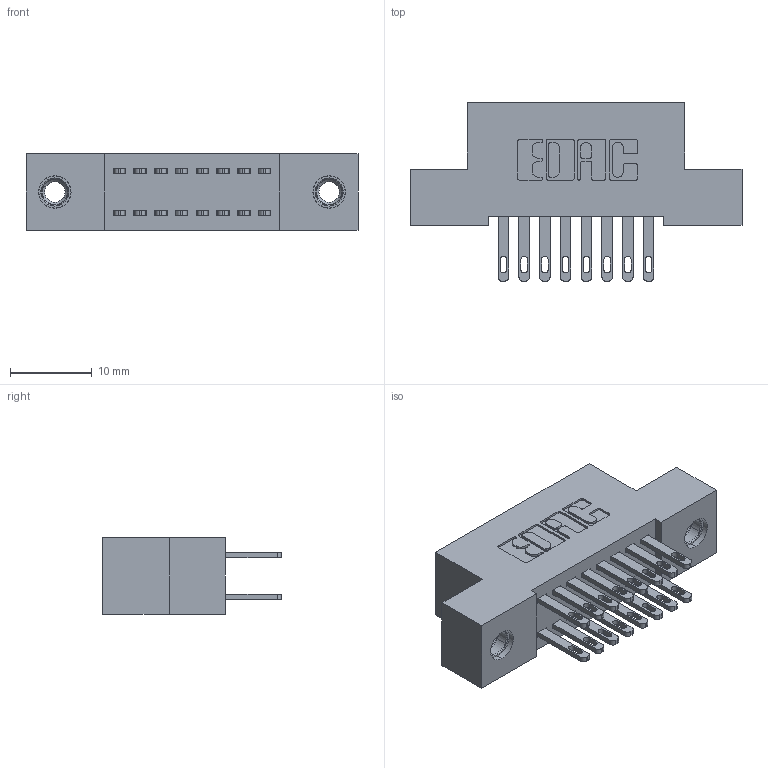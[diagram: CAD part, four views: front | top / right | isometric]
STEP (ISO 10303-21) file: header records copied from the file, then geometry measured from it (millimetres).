
FILE_DESCRIPTION (( 'STEP AP203' ), '1' );
FILE_NAME ('342-016-500-207.STEP', '2019-10-01T18:35:19', ( '' ), ( '' ), 'SwSTEP 2.0', 'SolidWorks 2016', '' );
FILE_SCHEMA (( 'CONFIG_CONTROL_DESIGN' ));
Length unit declared in the file: inch
Products named in the file (4): 345-292-001_345-293-100; 345-250-001_345-250-005-103; 342-016-500-207; 342 Part_TI
Assembly tree (19 placements, depth 2):
  342-016-500-207
    342 Part_TI
    345-292-001_345-293-100  x16
    345-250-001_345-250-005-103  x2
Bounding box: 40.64 x 21.85 x 9.4 mm (x, y, z)
Volume: 3526.8 mm3; surface area: 5081.9 mm2
Topology: 19 solids, 19 shells, 938 faces, 2787 edges, 1850 vertices
Faces by surface type: plane 578, cylinder 344, cone 12, torus 4
Entity records: 10528 total; most frequent: CARTESIAN_POINT 1765, ORIENTED_EDGE 1694, DIRECTION 1601, EDGE_CURVE 847, LINE 695, VECTOR 695, VERTEX_POINT 560, AXIS2_PLACEMENT_3D 453
